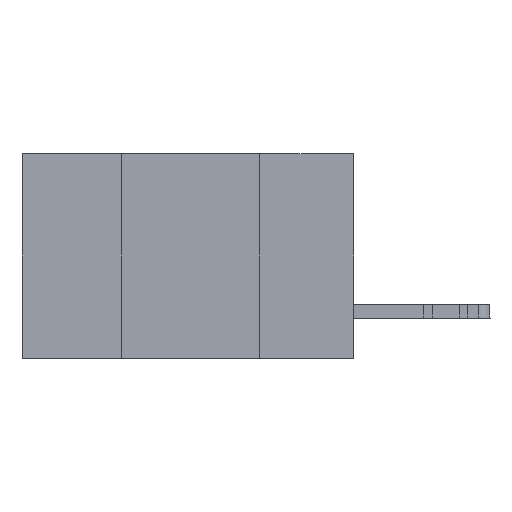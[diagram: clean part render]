
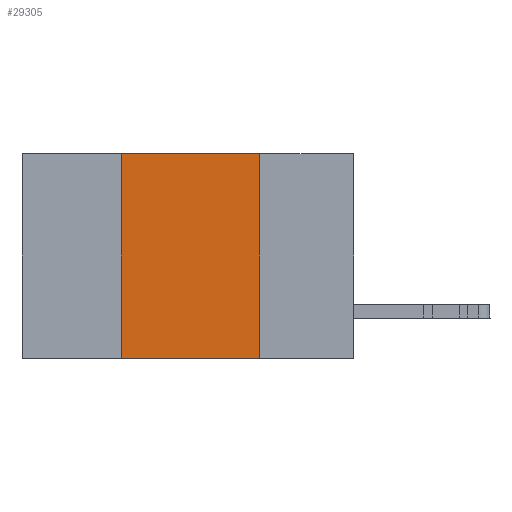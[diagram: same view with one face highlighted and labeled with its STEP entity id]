
A CAD part, left-side view. The second image highlights one B-rep face of the part: STEP entity #29305.
In plain terms, the highlighted planar face has unit normal (-1, 0, 0).
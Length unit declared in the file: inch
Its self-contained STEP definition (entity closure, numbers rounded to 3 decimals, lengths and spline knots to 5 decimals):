
#535 = LINE ( 'NONE', #12280, #28958 ) ;
#2412 = CARTESIAN_POINT ( 'NONE',  ( 0., 0.17, 0. ) ) ;
#4750 = LINE ( 'NONE', #34460, #16161 ) ;
#6011 = ORIENTED_EDGE ( 'NONE', *, *, #22405, .F. ) ;
#6257 = DIRECTION ( 'NONE',  ( 0., 0., -1. ) ) ;
#6851 = VERTEX_POINT ( 'NONE', #12138 ) ;
#7979 = VECTOR ( 'NONE', #41725, 39.37008 ) ;
#10046 = CARTESIAN_POINT ( 'NONE',  ( 0., 0.6, 0. ) ) ;
#11646 = FACE_OUTER_BOUND ( 'NONE', #13892, .T. ) ;
#12138 = CARTESIAN_POINT ( 'NONE',  ( 0., 0.42, 0. ) ) ;
#12280 = CARTESIAN_POINT ( 'NONE',  ( 0., 0.42, 0. ) ) ;
#13892 = EDGE_LOOP ( 'NONE', ( #6011, #39204, #19912, #28399 ) ) ;
#14256 = VERTEX_POINT ( 'NONE', #39982 ) ;
#14699 = DIRECTION ( 'NONE',  ( 0., -1., 0. ) ) ;
#15060 = EDGE_CURVE ( 'NONE', #14256, #16025, #4750, .T. ) ;
#15938 = AXIS2_PLACEMENT_3D ( 'NONE', #34390, #28513, #6257 ) ;
#16025 = VERTEX_POINT ( 'NONE', #28190 ) ;
#16161 = VECTOR ( 'NONE', #14699, 39.37008 ) ;
#16304 = LINE ( 'NONE', #2412, #7979 ) ;
#19912 = ORIENTED_EDGE ( 'NONE', *, *, #32333, .F. ) ;
#20987 = VECTOR ( 'NONE', #35912, 39.37008 ) ;
#21115 = PLANE ( 'NONE',  #15938 ) ;
#22405 = EDGE_CURVE ( 'NONE', #35672, #16025, #16304, .T. ) ;
#28190 = CARTESIAN_POINT ( 'NONE',  ( 0., 0.17, -0.37 ) ) ;
#28399 = ORIENTED_EDGE ( 'NONE', *, *, #15060, .T. ) ;
#28513 = DIRECTION ( 'NONE',  ( 1., 0., 0. ) ) ;
#28958 = VECTOR ( 'NONE', #38679, 39.37008 ) ;
#29305 = ADVANCED_FACE ( 'NONE', ( #11646 ), #21115, .F. ) ;
#32333 = EDGE_CURVE ( 'NONE', #14256, #6851, #535, .T. ) ;
#34390 = CARTESIAN_POINT ( 'NONE',  ( 0., 0.6, 0. ) ) ;
#34460 = CARTESIAN_POINT ( 'NONE',  ( 0., 0.6, -0.37 ) ) ;
#35672 = VERTEX_POINT ( 'NONE', #37883 ) ;
#35912 = DIRECTION ( 'NONE',  ( 0., -1., 0. ) ) ;
#37883 = CARTESIAN_POINT ( 'NONE',  ( 0., 0.17, 0. ) ) ;
#38679 = DIRECTION ( 'NONE',  ( 0., 0., 1. ) ) ;
#39085 = EDGE_CURVE ( 'NONE', #6851, #35672, #42742, .T. ) ;
#39204 = ORIENTED_EDGE ( 'NONE', *, *, #39085, .F. ) ;
#39982 = CARTESIAN_POINT ( 'NONE',  ( 0., 0.42, -0.37 ) ) ;
#41725 = DIRECTION ( 'NONE',  ( 0., 0., -1. ) ) ;
#42742 = LINE ( 'NONE', #10046, #20987 ) ;
